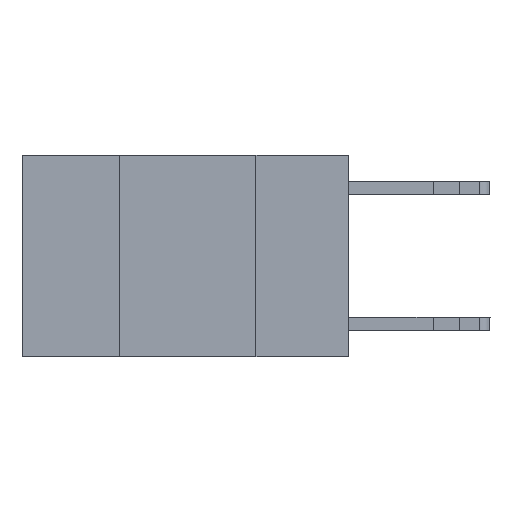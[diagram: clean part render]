
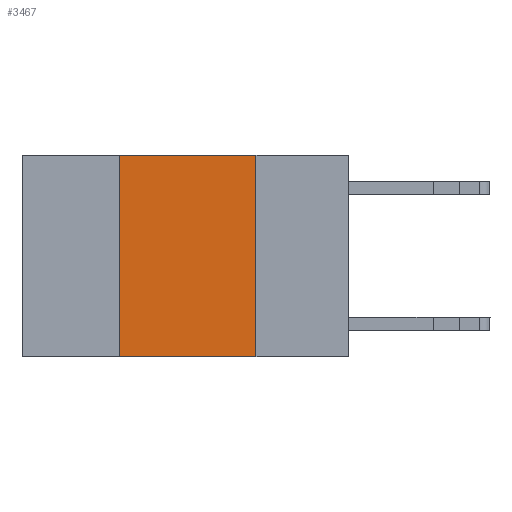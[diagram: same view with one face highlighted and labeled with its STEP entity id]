
A CAD part, left-side view. The second image highlights one B-rep face of the part: STEP entity #3467.
In plain terms, the highlighted planar face has unit normal (-1, 0, 0).
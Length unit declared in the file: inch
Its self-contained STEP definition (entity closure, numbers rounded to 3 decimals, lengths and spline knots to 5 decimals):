
#398 = DIRECTION ( 'NONE',  ( 0., 0., -1. ) ) ;
#1425 = DIRECTION ( 'NONE',  ( 0., -1., 0. ) ) ;
#1835 = VECTOR ( 'NONE', #1425, 39.37008 ) ;
#2917 = EDGE_CURVE ( 'NONE', #7954, #16478, #6408, .T. ) ;
#2983 = AXIS2_PLACEMENT_3D ( 'NONE', #15721, #8109, #14147 ) ;
#3350 = EDGE_CURVE ( 'NONE', #16478, #15574, #15041, .T. ) ;
#3437 = DIRECTION ( 'NONE',  ( 0., -1., 0. ) ) ;
#3467 = ADVANCED_FACE ( 'NONE', ( #9712 ), #5014, .F. ) ;
#3469 = EDGE_LOOP ( 'NONE', ( #18995, #13211, #7509, #18229 ) ) ;
#4985 = VECTOR ( 'NONE', #3437, 39.37008 ) ;
#5014 = PLANE ( 'NONE',  #2983 ) ;
#6408 = LINE ( 'NONE', #15595, #12040 ) ;
#6581 = LINE ( 'NONE', #17082, #4985 ) ;
#7509 = ORIENTED_EDGE ( 'NONE', *, *, #2917, .F. ) ;
#7954 = VERTEX_POINT ( 'NONE', #13358 ) ;
#8109 = DIRECTION ( 'NONE',  ( 1., 0., 0. ) ) ;
#9261 = VERTEX_POINT ( 'NONE', #17730 ) ;
#9515 = CARTESIAN_POINT ( 'NONE',  ( 0., 0.17, 0. ) ) ;
#9712 = FACE_OUTER_BOUND ( 'NONE', #3469, .T. ) ;
#10758 = EDGE_CURVE ( 'NONE', #7954, #9261, #6581, .T. ) ;
#11094 = LINE ( 'NONE', #9515, #15765 ) ;
#11691 = EDGE_CURVE ( 'NONE', #15574, #9261, #11094, .T. ) ;
#12040 = VECTOR ( 'NONE', #12743, 39.37008 ) ;
#12737 = CARTESIAN_POINT ( 'NONE',  ( 0., 0.42, 0. ) ) ;
#12743 = DIRECTION ( 'NONE',  ( 0., 0., 1. ) ) ;
#13211 = ORIENTED_EDGE ( 'NONE', *, *, #3350, .F. ) ;
#13358 = CARTESIAN_POINT ( 'NONE',  ( 0., 0.42, -0.37 ) ) ;
#14147 = DIRECTION ( 'NONE',  ( 0., 0., -1. ) ) ;
#15041 = LINE ( 'NONE', #17919, #1835 ) ;
#15470 = CARTESIAN_POINT ( 'NONE',  ( 0., 0.17, 0. ) ) ;
#15574 = VERTEX_POINT ( 'NONE', #15470 ) ;
#15595 = CARTESIAN_POINT ( 'NONE',  ( 0., 0.42, 0. ) ) ;
#15721 = CARTESIAN_POINT ( 'NONE',  ( 0., 0.6, 0. ) ) ;
#15765 = VECTOR ( 'NONE', #398, 39.37008 ) ;
#16478 = VERTEX_POINT ( 'NONE', #12737 ) ;
#17082 = CARTESIAN_POINT ( 'NONE',  ( 0., 0.6, -0.37 ) ) ;
#17730 = CARTESIAN_POINT ( 'NONE',  ( 0., 0.17, -0.37 ) ) ;
#17919 = CARTESIAN_POINT ( 'NONE',  ( 0., 0.6, 0. ) ) ;
#18229 = ORIENTED_EDGE ( 'NONE', *, *, #10758, .T. ) ;
#18995 = ORIENTED_EDGE ( 'NONE', *, *, #11691, .F. ) ;
